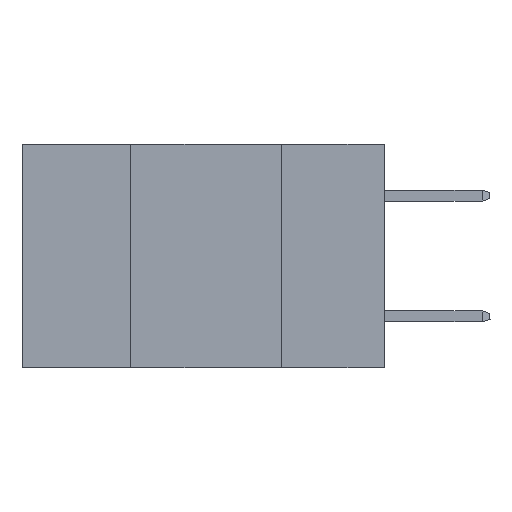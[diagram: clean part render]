
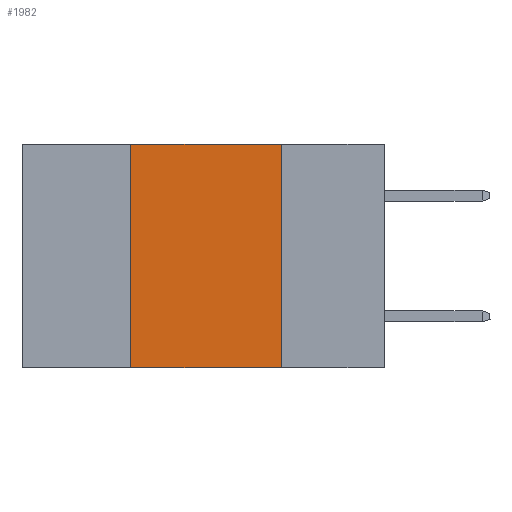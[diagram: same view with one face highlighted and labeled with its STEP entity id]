
A CAD part, left-side view. The second image highlights one B-rep face of the part: STEP entity #1982.
In plain terms, the highlighted planar face has unit normal (-1, 0, 0).
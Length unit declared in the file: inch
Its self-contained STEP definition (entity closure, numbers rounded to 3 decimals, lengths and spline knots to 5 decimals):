
#688 = DIRECTION ( 'NONE',  ( 0., 0., 1. ) ) ;
#1408 = VERTEX_POINT ( 'NONE', #14909 ) ;
#1958 = VERTEX_POINT ( 'NONE', #29586 ) ;
#1982 = ADVANCED_FACE ( 'NONE', ( #20724 ), #29774, .F. ) ;
#2836 = LINE ( 'NONE', #13709, #11377 ) ;
#4915 = CARTESIAN_POINT ( 'NONE',  ( 0., 0.6, 0. ) ) ;
#7550 = ORIENTED_EDGE ( 'NONE', *, *, #21089, .T. ) ;
#8614 = VECTOR ( 'NONE', #26732, 39.37008 ) ;
#10681 = VERTEX_POINT ( 'NONE', #11872 ) ;
#11377 = VECTOR ( 'NONE', #688, 39.37008 ) ;
#11626 = VERTEX_POINT ( 'NONE', #30684 ) ;
#11872 = CARTESIAN_POINT ( 'NONE',  ( 0., 0.42, -0.37 ) ) ;
#13085 = LINE ( 'NONE', #22244, #25848 ) ;
#13296 = EDGE_LOOP ( 'NONE', ( #20420, #15235, #29178, #7550 ) ) ;
#13709 = CARTESIAN_POINT ( 'NONE',  ( 0., 0.42, 0. ) ) ;
#14482 = EDGE_CURVE ( 'NONE', #11626, #1958, #13085, .T. ) ;
#14909 = CARTESIAN_POINT ( 'NONE',  ( 0., 0.42, 0. ) ) ;
#15235 = ORIENTED_EDGE ( 'NONE', *, *, #20065, .F. ) ;
#17104 = AXIS2_PLACEMENT_3D ( 'NONE', #32704, #27939, #27900 ) ;
#20065 = EDGE_CURVE ( 'NONE', #1408, #11626, #27102, .T. ) ;
#20420 = ORIENTED_EDGE ( 'NONE', *, *, #14482, .F. ) ;
#20724 = FACE_OUTER_BOUND ( 'NONE', #13296, .T. ) ;
#21089 = EDGE_CURVE ( 'NONE', #10681, #1958, #22272, .T. ) ;
#22244 = CARTESIAN_POINT ( 'NONE',  ( 0., 0.17, 0. ) ) ;
#22272 = LINE ( 'NONE', #24197, #8614 ) ;
#22920 = DIRECTION ( 'NONE',  ( 0., -1., 0. ) ) ;
#24197 = CARTESIAN_POINT ( 'NONE',  ( 0., 0.6, -0.37 ) ) ;
#24792 = DIRECTION ( 'NONE',  ( 0., 0., -1. ) ) ;
#25362 = EDGE_CURVE ( 'NONE', #10681, #1408, #2836, .T. ) ;
#25848 = VECTOR ( 'NONE', #24792, 39.37008 ) ;
#26732 = DIRECTION ( 'NONE',  ( 0., -1., 0. ) ) ;
#27102 = LINE ( 'NONE', #4915, #27878 ) ;
#27878 = VECTOR ( 'NONE', #22920, 39.37008 ) ;
#27900 = DIRECTION ( 'NONE',  ( 0., 0., -1. ) ) ;
#27939 = DIRECTION ( 'NONE',  ( 1., 0., 0. ) ) ;
#29178 = ORIENTED_EDGE ( 'NONE', *, *, #25362, .F. ) ;
#29586 = CARTESIAN_POINT ( 'NONE',  ( 0., 0.17, -0.37 ) ) ;
#29774 = PLANE ( 'NONE',  #17104 ) ;
#30684 = CARTESIAN_POINT ( 'NONE',  ( 0., 0.17, 0. ) ) ;
#32704 = CARTESIAN_POINT ( 'NONE',  ( 0., 0.6, 0. ) ) ;
